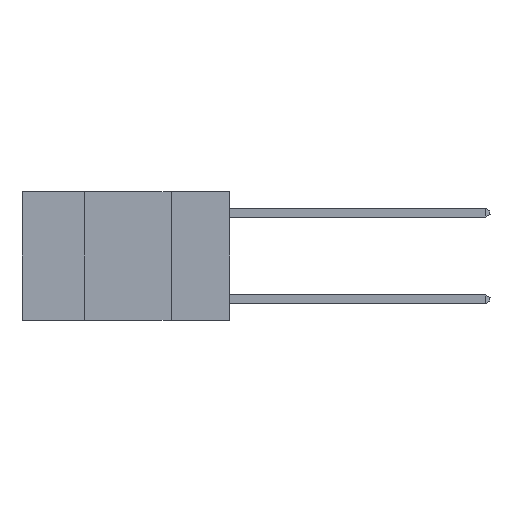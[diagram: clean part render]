
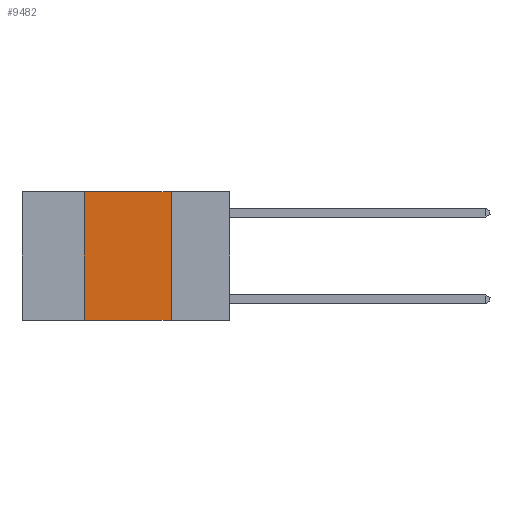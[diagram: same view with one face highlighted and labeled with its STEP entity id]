
A CAD part, left-side view. The second image highlights one B-rep face of the part: STEP entity #9482.
In plain terms, the highlighted planar face has unit normal (-1, 0, 0).
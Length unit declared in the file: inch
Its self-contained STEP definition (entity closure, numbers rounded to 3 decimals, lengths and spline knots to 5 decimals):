
#507 = CARTESIAN_POINT ( 'NONE',  ( 0., 0.6, -0.37 ) ) ;
#907 = DIRECTION ( 'NONE',  ( 1., 0., 0. ) ) ;
#1262 = VERTEX_POINT ( 'NONE', #7287 ) ;
#1431 = CARTESIAN_POINT ( 'NONE',  ( 0., 0.42, 0. ) ) ;
#1803 = CARTESIAN_POINT ( 'NONE',  ( 0., 0.42, -0.37 ) ) ;
#2731 = AXIS2_PLACEMENT_3D ( 'NONE', #13576, #907, #3668 ) ;
#2756 = ORIENTED_EDGE ( 'NONE', *, *, #7245, .F. ) ;
#3024 = VECTOR ( 'NONE', #6410, 39.37008 ) ;
#3048 = VERTEX_POINT ( 'NONE', #11235 ) ;
#3668 = DIRECTION ( 'NONE',  ( 0., 0., -1. ) ) ;
#4789 = CARTESIAN_POINT ( 'NONE',  ( 0., 0.17, 0. ) ) ;
#5786 = CARTESIAN_POINT ( 'NONE',  ( 0., 0.17, 0. ) ) ;
#6005 = LINE ( 'NONE', #4789, #9440 ) ;
#6040 = EDGE_CURVE ( 'NONE', #9367, #1262, #11343, .T. ) ;
#6402 = ORIENTED_EDGE ( 'NONE', *, *, #13547, .F. ) ;
#6410 = DIRECTION ( 'NONE',  ( 0., 0., 1. ) ) ;
#6545 = LINE ( 'NONE', #11319, #9883 ) ;
#7112 = ORIENTED_EDGE ( 'NONE', *, *, #9342, .T. ) ;
#7245 = EDGE_CURVE ( 'NONE', #11211, #3048, #6005, .T. ) ;
#7287 = CARTESIAN_POINT ( 'NONE',  ( 0., 0.42, 0. ) ) ;
#7352 = FACE_OUTER_BOUND ( 'NONE', #15038, .T. ) ;
#8234 = ORIENTED_EDGE ( 'NONE', *, *, #6040, .F. ) ;
#9140 = DIRECTION ( 'NONE',  ( 0., -1., 0. ) ) ;
#9342 = EDGE_CURVE ( 'NONE', #9367, #3048, #11898, .T. ) ;
#9367 = VERTEX_POINT ( 'NONE', #1803 ) ;
#9440 = VECTOR ( 'NONE', #14780, 39.37008 ) ;
#9450 = DIRECTION ( 'NONE',  ( 0., -1., 0. ) ) ;
#9482 = ADVANCED_FACE ( 'NONE', ( #7352 ), #9920, .F. ) ;
#9883 = VECTOR ( 'NONE', #9140, 39.37008 ) ;
#9920 = PLANE ( 'NONE',  #2731 ) ;
#11211 = VERTEX_POINT ( 'NONE', #5786 ) ;
#11235 = CARTESIAN_POINT ( 'NONE',  ( 0., 0.17, -0.37 ) ) ;
#11319 = CARTESIAN_POINT ( 'NONE',  ( 0., 0.6, 0. ) ) ;
#11343 = LINE ( 'NONE', #1431, #3024 ) ;
#11898 = LINE ( 'NONE', #507, #12940 ) ;
#12940 = VECTOR ( 'NONE', #9450, 39.37008 ) ;
#13547 = EDGE_CURVE ( 'NONE', #1262, #11211, #6545, .T. ) ;
#13576 = CARTESIAN_POINT ( 'NONE',  ( 0., 0.6, 0. ) ) ;
#14780 = DIRECTION ( 'NONE',  ( 0., 0., -1. ) ) ;
#15038 = EDGE_LOOP ( 'NONE', ( #2756, #6402, #8234, #7112 ) ) ;
